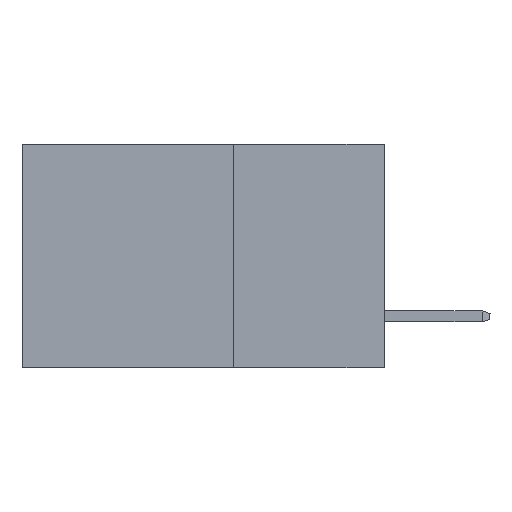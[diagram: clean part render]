
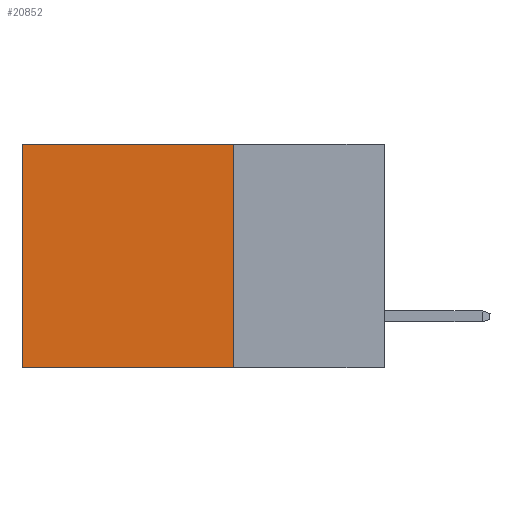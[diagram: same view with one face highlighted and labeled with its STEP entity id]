
A CAD part, left-side view. The second image highlights one B-rep face of the part: STEP entity #20852.
In plain terms, the highlighted planar face has unit normal (-1, 0, 0).
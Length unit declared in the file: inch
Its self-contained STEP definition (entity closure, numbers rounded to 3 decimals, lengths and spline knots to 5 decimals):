
#734 = EDGE_CURVE ( 'NONE', #24650, #970, #13828, .T. ) ;
#970 = VERTEX_POINT ( 'NONE', #6677 ) ;
#1279 = CARTESIAN_POINT ( 'NONE',  ( 0.2615, 0.25, -0.37 ) ) ;
#1786 = EDGE_CURVE ( 'NONE', #10045, #14869, #18049, .T. ) ;
#2479 = EDGE_CURVE ( 'NONE', #970, #14869, #14917, .T. ) ;
#2481 = CARTESIAN_POINT ( 'NONE',  ( 0.2615, 0.25, -0.37 ) ) ;
#2970 = FACE_OUTER_BOUND ( 'NONE', #8025, .T. ) ;
#4297 = DIRECTION ( 'NONE',  ( 0., 1., 0. ) ) ;
#4619 = DIRECTION ( 'NONE',  ( 0., 1., 0. ) ) ;
#6677 = CARTESIAN_POINT ( 'NONE',  ( 0.2615, 0.6, 0. ) ) ;
#7072 = VECTOR ( 'NONE', #4619, 39.37008 ) ;
#8025 = EDGE_LOOP ( 'NONE', ( #19057, #19257, #9176, #14398 ) ) ;
#8617 = DIRECTION ( 'NONE',  ( 1., 0., 0. ) ) ;
#9169 = LINE ( 'NONE', #12939, #15388 ) ;
#9176 = ORIENTED_EDGE ( 'NONE', *, *, #18692, .F. ) ;
#9428 = AXIS2_PLACEMENT_3D ( 'NONE', #22275, #8617, #12751 ) ;
#10045 = VERTEX_POINT ( 'NONE', #1279 ) ;
#10595 = CARTESIAN_POINT ( 'NONE',  ( 0.2615, 0.6, -0.37 ) ) ;
#10987 = PLANE ( 'NONE',  #9428 ) ;
#12751 = DIRECTION ( 'NONE',  ( 0., 0., -1. ) ) ;
#12939 = CARTESIAN_POINT ( 'NONE',  ( 0.2615, 0.25, -0.37 ) ) ;
#13828 = LINE ( 'NONE', #17850, #22902 ) ;
#14398 = ORIENTED_EDGE ( 'NONE', *, *, #734, .T. ) ;
#14869 = VERTEX_POINT ( 'NONE', #10595 ) ;
#14917 = LINE ( 'NONE', #24673, #16785 ) ;
#15388 = VECTOR ( 'NONE', #20590, 39.37008 ) ;
#16785 = VECTOR ( 'NONE', #22788, 39.37008 ) ;
#17850 = CARTESIAN_POINT ( 'NONE',  ( 0.2615, 0.25, 0. ) ) ;
#18049 = LINE ( 'NONE', #2481, #7072 ) ;
#18692 = EDGE_CURVE ( 'NONE', #24650, #10045, #9169, .T. ) ;
#19057 = ORIENTED_EDGE ( 'NONE', *, *, #2479, .T. ) ;
#19257 = ORIENTED_EDGE ( 'NONE', *, *, #1786, .F. ) ;
#20310 = CARTESIAN_POINT ( 'NONE',  ( 0.2615, 0.25, 0. ) ) ;
#20590 = DIRECTION ( 'NONE',  ( 0., 0., -1. ) ) ;
#20852 = ADVANCED_FACE ( 'NONE', ( #2970 ), #10987, .F. ) ;
#22275 = CARTESIAN_POINT ( 'NONE',  ( 0.2615, 0.25, -0.37 ) ) ;
#22788 = DIRECTION ( 'NONE',  ( 0., 0., -1. ) ) ;
#22902 = VECTOR ( 'NONE', #4297, 39.37008 ) ;
#24650 = VERTEX_POINT ( 'NONE', #20310 ) ;
#24673 = CARTESIAN_POINT ( 'NONE',  ( 0.2615, 0.6, -0.37 ) ) ;
